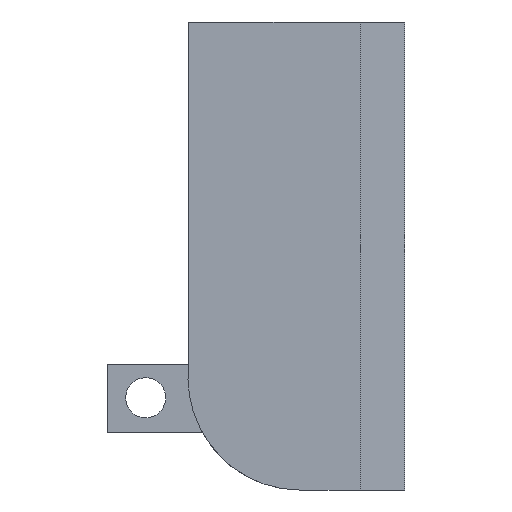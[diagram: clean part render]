
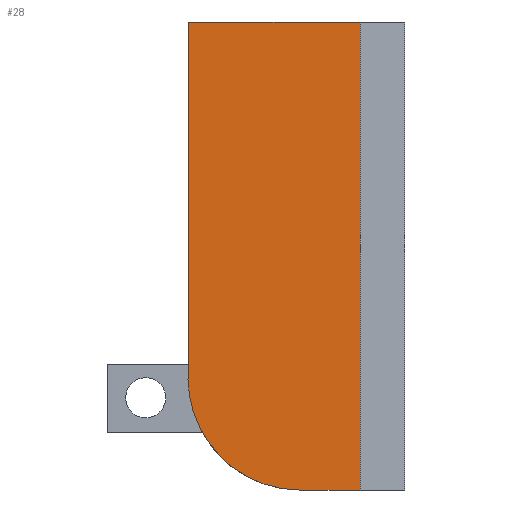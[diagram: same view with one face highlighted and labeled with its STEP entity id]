
A CAD part, front view. The second image highlights one B-rep face of the part: STEP entity #28.
In plain terms, the highlighted planar face has unit normal (0, -1, 0).
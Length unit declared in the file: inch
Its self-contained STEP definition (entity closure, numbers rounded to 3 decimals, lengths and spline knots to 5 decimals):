
#6 = EDGE_CURVE ( 'NONE', #708, #673, #761, .T. ) ;
#18 = FACE_OUTER_BOUND ( 'NONE', #426, .T. ) ;
#28 = ADVANCED_FACE ( 'NONE', ( #18 ), #343, .T. ) ;
#51 = LINE ( 'NONE', #188, #557 ) ;
#53 = ORIENTED_EDGE ( 'NONE', *, *, #211, .F. ) ;
#78 = CARTESIAN_POINT ( 'NONE',  ( 1.16, 0., 0. ) ) ;
#82 = EDGE_CURVE ( 'NONE', #731, #449, #51, .T. ) ;
#84 = ORIENTED_EDGE ( 'NONE', *, *, #719, .T. ) ;
#97 = ORIENTED_EDGE ( 'NONE', *, *, #82, .T. ) ;
#147 = DIRECTION ( 'NONE',  ( 0., -1., 0. ) ) ;
#154 = DIRECTION ( 'NONE',  ( 0., -1., 0. ) ) ;
#164 = CARTESIAN_POINT ( 'NONE',  ( 0., 0., 0. ) ) ;
#188 = CARTESIAN_POINT ( 'NONE',  ( 0., 0., -4.33877 ) ) ;
#207 = CARTESIAN_POINT ( 'NONE',  ( 0., 0., -6.65 ) ) ;
#208 = LINE ( 'NONE', #224, #488 ) ;
#211 = EDGE_CURVE ( 'NONE', #744, #449, #208, .T. ) ;
#219 = CARTESIAN_POINT ( 'NONE',  ( 0.75, 0., -6.75 ) ) ;
#224 = CARTESIAN_POINT ( 'NONE',  ( 0., 0., 0. ) ) ;
#236 = VERTEX_POINT ( 'NONE', #468 ) ;
#243 = CIRCLE ( 'NONE', #741, 0.75 ) ;
#263 = AXIS2_PLACEMENT_3D ( 'NONE', #688, #147, #325 ) ;
#282 = CARTESIAN_POINT ( 'NONE',  ( 0., 0., -7.5 ) ) ;
#289 = DIRECTION ( 'NONE',  ( 0., -1., 0. ) ) ;
#311 = VECTOR ( 'NONE', #502, 39.37008 ) ;
#325 = DIRECTION ( 'NONE',  ( 0., 0., -1. ) ) ;
#340 = DIRECTION ( 'NONE',  ( -1., 0., 0. ) ) ;
#343 = PLANE ( 'NONE',  #406 ) ;
#355 = CARTESIAN_POINT ( 'NONE',  ( 0.75, 0., -7.5 ) ) ;
#376 = CARTESIAN_POINT ( 'NONE',  ( 1.16, 0., -4.33877 ) ) ;
#384 = CARTESIAN_POINT ( 'NONE',  ( 0., 0., -4.33877 ) ) ;
#406 = AXIS2_PLACEMENT_3D ( 'NONE', #164, #154, #462 ) ;
#413 = DIRECTION ( 'NONE',  ( 0., 0., -1. ) ) ;
#426 = EDGE_LOOP ( 'NONE', ( #649, #97, #53, #84, #500, #713 ) ) ;
#449 = VERTEX_POINT ( 'NONE', #384 ) ;
#450 = CIRCLE ( 'NONE', #263, 0.76722 ) ;
#462 = DIRECTION ( 'NONE',  ( 0., 0., -1. ) ) ;
#467 = EDGE_CURVE ( 'NONE', #236, #673, #243, .T. ) ;
#468 = CARTESIAN_POINT ( 'NONE',  ( 0.06707, 0., -7.06 ) ) ;
#488 = VECTOR ( 'NONE', #533, 39.37008 ) ;
#500 = ORIENTED_EDGE ( 'NONE', *, *, #467, .T. ) ;
#502 = DIRECTION ( 'NONE',  ( 0., 0., 1. ) ) ;
#533 = DIRECTION ( 'NONE',  ( 0., 0., 1. ) ) ;
#557 = VECTOR ( 'NONE', #617, 39.37008 ) ;
#596 = VECTOR ( 'NONE', #340, 39.37008 ) ;
#617 = DIRECTION ( 'NONE',  ( -1., 0., 0. ) ) ;
#638 = LINE ( 'NONE', #78, #311 ) ;
#649 = ORIENTED_EDGE ( 'NONE', *, *, #763, .T. ) ;
#671 = CARTESIAN_POINT ( 'NONE',  ( 1.16, 0., -7.5 ) ) ;
#673 = VERTEX_POINT ( 'NONE', #355 ) ;
#688 = CARTESIAN_POINT ( 'NONE',  ( 0.76241, 0., -6.73577 ) ) ;
#708 = VERTEX_POINT ( 'NONE', #671 ) ;
#713 = ORIENTED_EDGE ( 'NONE', *, *, #6, .F. ) ;
#719 = EDGE_CURVE ( 'NONE', #744, #236, #450, .T. ) ;
#731 = VERTEX_POINT ( 'NONE', #376 ) ;
#741 = AXIS2_PLACEMENT_3D ( 'NONE', #219, #289, #413 ) ;
#744 = VERTEX_POINT ( 'NONE', #207 ) ;
#761 = LINE ( 'NONE', #282, #596 ) ;
#763 = EDGE_CURVE ( 'NONE', #708, #731, #638, .T. ) ;
